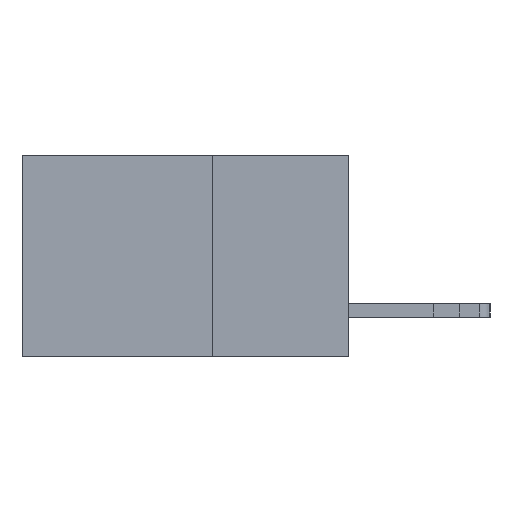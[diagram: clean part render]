
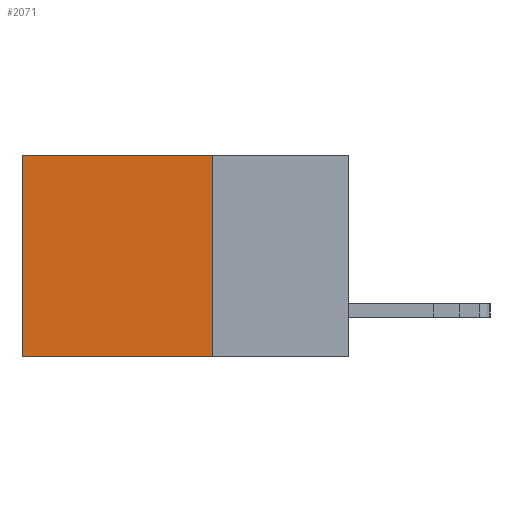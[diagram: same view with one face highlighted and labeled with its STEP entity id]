
A CAD part, left-side view. The second image highlights one B-rep face of the part: STEP entity #2071.
In plain terms, the highlighted planar face has unit normal (-1, 0, 0).
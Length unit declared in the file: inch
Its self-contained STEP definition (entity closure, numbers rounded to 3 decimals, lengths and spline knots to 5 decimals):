
#471 = CARTESIAN_POINT ( 'NONE',  ( 0.2615, 0.25, 0. ) ) ;
#651 = LINE ( 'NONE', #9010, #1154 ) ;
#674 = EDGE_CURVE ( 'NONE', #3520, #7251, #6707, .T. ) ;
#1154 = VECTOR ( 'NONE', #12401, 39.37008 ) ;
#2071 = ADVANCED_FACE ( 'NONE', ( #4375 ), #19936, .F. ) ;
#3045 = DIRECTION ( 'NONE',  ( 0., 1., 0. ) ) ;
#3499 = LINE ( 'NONE', #19366, #12508 ) ;
#3520 = VERTEX_POINT ( 'NONE', #5490 ) ;
#3908 = CARTESIAN_POINT ( 'NONE',  ( 0.2615, 0.25, -0.37 ) ) ;
#4375 = FACE_OUTER_BOUND ( 'NONE', #7462, .T. ) ;
#4594 = ORIENTED_EDGE ( 'NONE', *, *, #18920, .T. ) ;
#5192 = CARTESIAN_POINT ( 'NONE',  ( 0.2615, 0.6, 0. ) ) ;
#5490 = CARTESIAN_POINT ( 'NONE',  ( 0.2615, 0.25, -0.37 ) ) ;
#6707 = LINE ( 'NONE', #3908, #10675 ) ;
#7251 = VERTEX_POINT ( 'NONE', #9453 ) ;
#7462 = EDGE_LOOP ( 'NONE', ( #4594, #10900, #14617, #10300 ) ) ;
#9010 = CARTESIAN_POINT ( 'NONE',  ( 0.2615, 0.25, 0. ) ) ;
#9425 = DIRECTION ( 'NONE',  ( 0., 0., -1. ) ) ;
#9453 = CARTESIAN_POINT ( 'NONE',  ( 0.2615, 0.6, -0.37 ) ) ;
#10300 = ORIENTED_EDGE ( 'NONE', *, *, #11898, .T. ) ;
#10675 = VECTOR ( 'NONE', #3045, 39.37008 ) ;
#10900 = ORIENTED_EDGE ( 'NONE', *, *, #674, .F. ) ;
#11898 = EDGE_CURVE ( 'NONE', #13194, #20664, #651, .T. ) ;
#12279 = CARTESIAN_POINT ( 'NONE',  ( 0.2615, 0.25, -0.37 ) ) ;
#12401 = DIRECTION ( 'NONE',  ( 0., 1., 0. ) ) ;
#12508 = VECTOR ( 'NONE', #9425, 39.37008 ) ;
#13194 = VERTEX_POINT ( 'NONE', #471 ) ;
#13249 = EDGE_CURVE ( 'NONE', #13194, #3520, #17329, .T. ) ;
#14617 = ORIENTED_EDGE ( 'NONE', *, *, #13249, .F. ) ;
#17293 = DIRECTION ( 'NONE',  ( 0., 0., -1. ) ) ;
#17329 = LINE ( 'NONE', #12279, #21096 ) ;
#17446 = AXIS2_PLACEMENT_3D ( 'NONE', #19911, #19890, #19888 ) ;
#18920 = EDGE_CURVE ( 'NONE', #20664, #7251, #3499, .T. ) ;
#19366 = CARTESIAN_POINT ( 'NONE',  ( 0.2615, 0.6, -0.37 ) ) ;
#19888 = DIRECTION ( 'NONE',  ( 0., 0., -1. ) ) ;
#19890 = DIRECTION ( 'NONE',  ( 1., 0., 0. ) ) ;
#19911 = CARTESIAN_POINT ( 'NONE',  ( 0.2615, 0.25, -0.37 ) ) ;
#19936 = PLANE ( 'NONE',  #17446 ) ;
#20664 = VERTEX_POINT ( 'NONE', #5192 ) ;
#21096 = VECTOR ( 'NONE', #17293, 39.37008 ) ;
